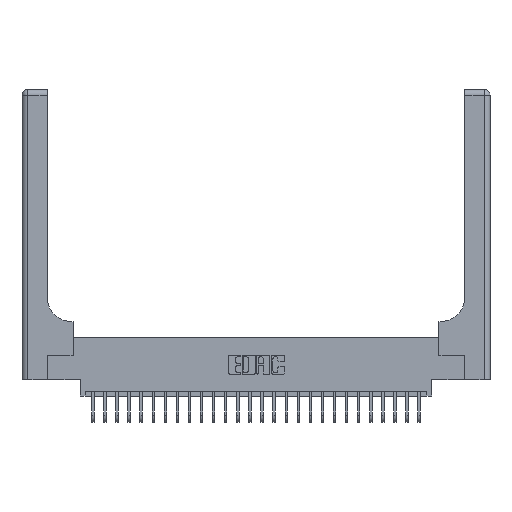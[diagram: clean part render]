
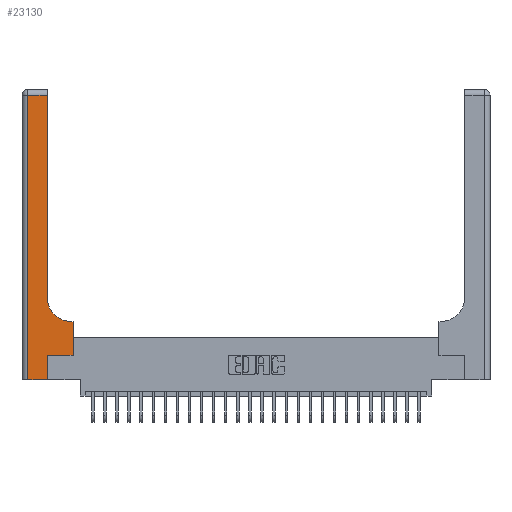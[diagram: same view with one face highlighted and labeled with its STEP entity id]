
A CAD part, top view. The second image highlights one B-rep face of the part: STEP entity #23130.
In plain terms, the highlighted planar face has unit normal (0, 0, 1).
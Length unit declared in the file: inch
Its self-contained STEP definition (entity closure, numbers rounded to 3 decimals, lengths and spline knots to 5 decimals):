
#119 = VERTEX_POINT ( 'NONE', #23997 ) ;
#724 = LINE ( 'NONE', #21075, #18752 ) ;
#756 = CARTESIAN_POINT ( 'NONE',  ( 0.26, 3., 0.37 ) ) ;
#1033 = LINE ( 'NONE', #16924, #2615 ) ;
#1154 = VERTEX_POINT ( 'NONE', #16690 ) ;
#1537 = ORIENTED_EDGE ( 'NONE', *, *, #17360, .T. ) ;
#1571 = EDGE_CURVE ( 'NONE', #15986, #21559, #1033, .T. ) ;
#1884 = VECTOR ( 'NONE', #21268, 39.37008 ) ;
#1957 = ORIENTED_EDGE ( 'NONE', *, *, #20328, .T. ) ;
#2320 = EDGE_CURVE ( 'NONE', #119, #17707, #24210, .T. ) ;
#2408 = VECTOR ( 'NONE', #24437, 39.37008 ) ;
#2422 = ORIENTED_EDGE ( 'NONE', *, *, #2320, .T. ) ;
#2615 = VECTOR ( 'NONE', #3084, 39.37008 ) ;
#2679 = CARTESIAN_POINT ( 'NONE',  ( 0.265, 0.25, 0.37 ) ) ;
#3084 = DIRECTION ( 'NONE',  ( 0., 1., 0. ) ) ;
#3378 = CARTESIAN_POINT ( 'NONE',  ( 0.265, 0., 0.37 ) ) ;
#4275 = VERTEX_POINT ( 'NONE', #12065 ) ;
#4968 = DIRECTION ( 'NONE',  ( 1., 0., 0. ) ) ;
#5074 = DIRECTION ( 'NONE',  ( 0., 1., 0. ) ) ;
#5110 = DIRECTION ( 'NONE',  ( 0., 0., -1. ) ) ;
#5780 = CARTESIAN_POINT ( 'NONE',  ( 0.06, 3., 0.37 ) ) ;
#6216 = VECTOR ( 'NONE', #22171, 39.37008 ) ;
#6279 = DIRECTION ( 'NONE',  ( 0., -1., 0. ) ) ;
#6881 = CARTESIAN_POINT ( 'NONE',  ( 0., 0., 0.37 ) ) ;
#7023 = ORIENTED_EDGE ( 'NONE', *, *, #18320, .T. ) ;
#8602 = ORIENTED_EDGE ( 'NONE', *, *, #24795, .T. ) ;
#10362 = AXIS2_PLACEMENT_3D ( 'NONE', #17428, #15516, #19198 ) ;
#11277 = LINE ( 'NONE', #19026, #1884 ) ;
#11895 = EDGE_CURVE ( 'NONE', #17192, #18852, #18736, .T. ) ;
#12065 = CARTESIAN_POINT ( 'NONE',  ( 0.51, 0.6, 0.37 ) ) ;
#12539 = CARTESIAN_POINT ( 'NONE',  ( 0.06, 2.94, 0.37 ) ) ;
#12629 = ORIENTED_EDGE ( 'NONE', *, *, #18781, .T. ) ;
#12643 = VECTOR ( 'NONE', #6279, 39.37008 ) ;
#12811 = CIRCLE ( 'NONE', #10362, 0.25 ) ;
#13229 = FACE_OUTER_BOUND ( 'NONE', #23704, .T. ) ;
#14798 = ORIENTED_EDGE ( 'NONE', *, *, #11895, .T. ) ;
#15010 = PLANE ( 'NONE',  #17228 ) ;
#15431 = LINE ( 'NONE', #5780, #12643 ) ;
#15516 = DIRECTION ( 'NONE',  ( 0., 0., -1. ) ) ;
#15986 = VERTEX_POINT ( 'NONE', #23337 ) ;
#16007 = LINE ( 'NONE', #756, #24410 ) ;
#16690 = CARTESIAN_POINT ( 'NONE',  ( 0.26, 0.85, 0.37 ) ) ;
#16761 = LINE ( 'NONE', #6881, #24361 ) ;
#16924 = CARTESIAN_POINT ( 'NONE',  ( 0.528, 0.25, 0.37 ) ) ;
#16960 = CARTESIAN_POINT ( 'NONE',  ( 0., 2.94, 0.37 ) ) ;
#17192 = VERTEX_POINT ( 'NONE', #19684 ) ;
#17228 = AXIS2_PLACEMENT_3D ( 'NONE', #21059, #5110, #20945 ) ;
#17360 = EDGE_CURVE ( 'NONE', #19210, #17192, #16761, .T. ) ;
#17428 = CARTESIAN_POINT ( 'NONE',  ( 0.51, 0.85, 0.37 ) ) ;
#17707 = VERTEX_POINT ( 'NONE', #12539 ) ;
#18320 = EDGE_CURVE ( 'NONE', #17707, #19210, #15431, .T. ) ;
#18736 = LINE ( 'NONE', #3378, #2408 ) ;
#18752 = VECTOR ( 'NONE', #21788, 39.37008 ) ;
#18781 = EDGE_CURVE ( 'NONE', #1154, #119, #16007, .T. ) ;
#18791 = ORIENTED_EDGE ( 'NONE', *, *, #24058, .T. ) ;
#18852 = VERTEX_POINT ( 'NONE', #2679 ) ;
#19026 = CARTESIAN_POINT ( 'NONE',  ( 0.265, 0.25, 0.37 ) ) ;
#19095 = ORIENTED_EDGE ( 'NONE', *, *, #1571, .T. ) ;
#19198 = DIRECTION ( 'NONE',  ( 1., 0., 0. ) ) ;
#19210 = VERTEX_POINT ( 'NONE', #19877 ) ;
#19324 = CARTESIAN_POINT ( 'NONE',  ( 0.528, 0.6, 0.37 ) ) ;
#19684 = CARTESIAN_POINT ( 'NONE',  ( 0.265, 0., 0.37 ) ) ;
#19877 = CARTESIAN_POINT ( 'NONE',  ( 0.06, 0., 0.37 ) ) ;
#20328 = EDGE_CURVE ( 'NONE', #21559, #4275, #724, .T. ) ;
#20945 = DIRECTION ( 'NONE',  ( -1., 0., 0. ) ) ;
#21059 = CARTESIAN_POINT ( 'NONE',  ( 0., 3., 0.37 ) ) ;
#21075 = CARTESIAN_POINT ( 'NONE',  ( 0.26, 0.6, 0.37 ) ) ;
#21268 = DIRECTION ( 'NONE',  ( 1., 0., 0. ) ) ;
#21559 = VERTEX_POINT ( 'NONE', #19324 ) ;
#21788 = DIRECTION ( 'NONE',  ( -1., 0., 0. ) ) ;
#22171 = DIRECTION ( 'NONE',  ( -1., 0., 0. ) ) ;
#23130 = ADVANCED_FACE ( 'NONE', ( #13229 ), #15010, .F. ) ;
#23337 = CARTESIAN_POINT ( 'NONE',  ( 0.528, 0.25, 0.37 ) ) ;
#23704 = EDGE_LOOP ( 'NONE', ( #12629, #2422, #7023, #1537, #14798, #8602, #19095, #1957, #18791 ) ) ;
#23997 = CARTESIAN_POINT ( 'NONE',  ( 0.26, 2.94, 0.37 ) ) ;
#24058 = EDGE_CURVE ( 'NONE', #4275, #1154, #12811, .T. ) ;
#24210 = LINE ( 'NONE', #16960, #6216 ) ;
#24361 = VECTOR ( 'NONE', #4968, 39.37008 ) ;
#24410 = VECTOR ( 'NONE', #5074, 39.37008 ) ;
#24437 = DIRECTION ( 'NONE',  ( 0., 1., 0. ) ) ;
#24795 = EDGE_CURVE ( 'NONE', #18852, #15986, #11277, .T. ) ;
